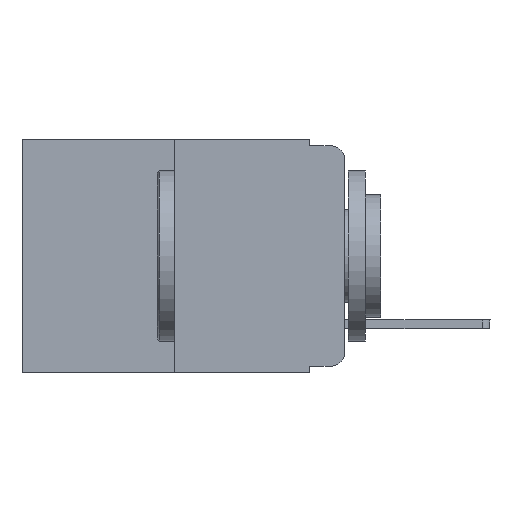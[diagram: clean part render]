
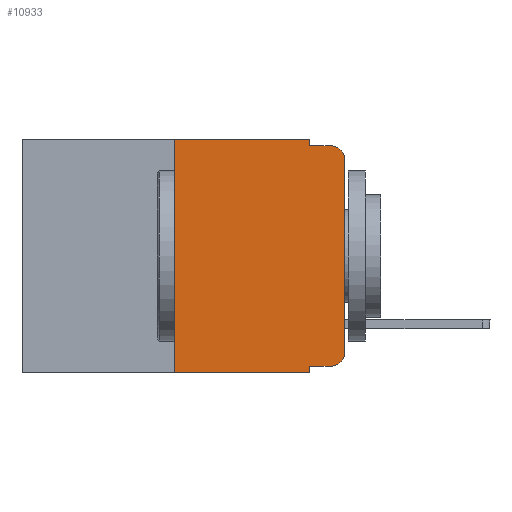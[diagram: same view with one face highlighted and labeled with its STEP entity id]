
A CAD part, left-side view. The second image highlights one B-rep face of the part: STEP entity #10933.
In plain terms, the highlighted planar face has unit normal (-1, 0, 0).
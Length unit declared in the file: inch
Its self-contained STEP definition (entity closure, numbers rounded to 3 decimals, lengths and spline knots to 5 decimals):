
#22 = CARTESIAN_POINT ( 'NONE',  ( 0., 0.051, -0.333 ) ) ;
#64 = DIRECTION ( 'NONE',  ( 0., 0., -1. ) ) ;
#146 = VECTOR ( 'NONE', #7066, 39.37008 ) ;
#222 = LINE ( 'NONE', #6759, #4909 ) ;
#269 = CARTESIAN_POINT ( 'NONE',  ( 0., 0.051, 0. ) ) ;
#316 = LINE ( 'NONE', #7918, #7166 ) ;
#426 = EDGE_CURVE ( 'NONE', #4306, #2158, #13773, .T. ) ;
#522 = CARTESIAN_POINT ( 'NONE',  ( 0., 0.02, -0.01 ) ) ;
#906 = CARTESIAN_POINT ( 'NONE',  ( 0., 0.25, 0. ) ) ;
#1368 = EDGE_LOOP ( 'NONE', ( #5111, #12547, #5237, #2367, #3803, #13229, #7071, #8952, #4279, #4212 ) ) ;
#1508 = VERTEX_POINT ( 'NONE', #906 ) ;
#1589 = LINE ( 'NONE', #14017, #3584 ) ;
#1869 = DIRECTION ( 'NONE',  ( -1., 0., 0. ) ) ;
#2158 = VERTEX_POINT ( 'NONE', #522 ) ;
#2354 = DIRECTION ( 'NONE',  ( 0., -1., 0. ) ) ;
#2367 = ORIENTED_EDGE ( 'NONE', *, *, #2426, .F. ) ;
#2403 = CIRCLE ( 'NONE', #7490, 0.02 ) ;
#2426 = EDGE_CURVE ( 'NONE', #7977, #4306, #222, .T. ) ;
#2478 = CARTESIAN_POINT ( 'NONE',  ( 0., 0., -0.03 ) ) ;
#2907 = DIRECTION ( 'NONE',  ( 0., 0., -1. ) ) ;
#3459 = LINE ( 'NONE', #269, #12423 ) ;
#3584 = VECTOR ( 'NONE', #5206, 39.37008 ) ;
#3803 = ORIENTED_EDGE ( 'NONE', *, *, #11077, .F. ) ;
#3999 = DIRECTION ( 'NONE',  ( 0., -1., 0. ) ) ;
#4024 = CARTESIAN_POINT ( 'NONE',  ( 0., 0.25, -0.343 ) ) ;
#4091 = EDGE_CURVE ( 'NONE', #8980, #8828, #10275, .T. ) ;
#4212 = ORIENTED_EDGE ( 'NONE', *, *, #5855, .T. ) ;
#4279 = ORIENTED_EDGE ( 'NONE', *, *, #4091, .T. ) ;
#4306 = VERTEX_POINT ( 'NONE', #5505 ) ;
#4570 = LINE ( 'NONE', #9970, #9867 ) ;
#4909 = VECTOR ( 'NONE', #64, 39.37008 ) ;
#5111 = ORIENTED_EDGE ( 'NONE', *, *, #8384, .T. ) ;
#5186 = VERTEX_POINT ( 'NONE', #2478 ) ;
#5206 = DIRECTION ( 'NONE',  ( 0., 0., 1. ) ) ;
#5237 = ORIENTED_EDGE ( 'NONE', *, *, #426, .F. ) ;
#5497 = AXIS2_PLACEMENT_3D ( 'NONE', #13297, #9700, #12213 ) ;
#5505 = CARTESIAN_POINT ( 'NONE',  ( 0., 0.051, -0.01 ) ) ;
#5759 = CARTESIAN_POINT ( 'NONE',  ( 0., 0.25, 0. ) ) ;
#5855 = EDGE_CURVE ( 'NONE', #8828, #12789, #2403, .T. ) ;
#6172 = CARTESIAN_POINT ( 'NONE',  ( 0., 0.051, -0.333 ) ) ;
#6341 = CARTESIAN_POINT ( 'NONE',  ( 0., 0., -0.313 ) ) ;
#6385 = DIRECTION ( 'NONE',  ( 1., 0., 0. ) ) ;
#6759 = CARTESIAN_POINT ( 'NONE',  ( 0., 0.051, 0. ) ) ;
#6895 = AXIS2_PLACEMENT_3D ( 'NONE', #10701, #6385, #2907 ) ;
#7066 = DIRECTION ( 'NONE',  ( 0., -1., 0. ) ) ;
#7071 = ORIENTED_EDGE ( 'NONE', *, *, #14133, .T. ) ;
#7166 = VECTOR ( 'NONE', #2354, 39.37008 ) ;
#7490 = AXIS2_PLACEMENT_3D ( 'NONE', #13669, #1869, #8530 ) ;
#7508 = EDGE_CURVE ( 'NONE', #12518, #1508, #7785, .T. ) ;
#7785 = LINE ( 'NONE', #5759, #12600 ) ;
#7918 = CARTESIAN_POINT ( 'NONE',  ( 0., 0.473, -0.343 ) ) ;
#7977 = VERTEX_POINT ( 'NONE', #9417 ) ;
#8284 = CARTESIAN_POINT ( 'NONE',  ( 0., 0.051, -0.01 ) ) ;
#8377 = VECTOR ( 'NONE', #3999, 39.37008 ) ;
#8384 = EDGE_CURVE ( 'NONE', #12789, #5186, #1589, .T. ) ;
#8530 = DIRECTION ( 'NONE',  ( 0., 0., -1. ) ) ;
#8538 = VERTEX_POINT ( 'NONE', #10906 ) ;
#8828 = VERTEX_POINT ( 'NONE', #12565 ) ;
#8952 = ORIENTED_EDGE ( 'NONE', *, *, #11555, .F. ) ;
#8980 = VERTEX_POINT ( 'NONE', #22 ) ;
#9417 = CARTESIAN_POINT ( 'NONE',  ( 0., 0.051, 0. ) ) ;
#9700 = DIRECTION ( 'NONE',  ( -1., 0., 0. ) ) ;
#9867 = VECTOR ( 'NONE', #14166, 39.37008 ) ;
#9970 = CARTESIAN_POINT ( 'NONE',  ( 0., 0.473, 0. ) ) ;
#10075 = DIRECTION ( 'NONE',  ( 0., 0., 1. ) ) ;
#10275 = LINE ( 'NONE', #6172, #8377 ) ;
#10701 = CARTESIAN_POINT ( 'NONE',  ( 0., 0.473, 0. ) ) ;
#10906 = CARTESIAN_POINT ( 'NONE',  ( 0., 0.051, -0.343 ) ) ;
#10933 = ADVANCED_FACE ( 'NONE', ( #14024 ), #14099, .F. ) ;
#11077 = EDGE_CURVE ( 'NONE', #1508, #7977, #4570, .T. ) ;
#11162 = EDGE_CURVE ( 'NONE', #5186, #2158, #13572, .T. ) ;
#11555 = EDGE_CURVE ( 'NONE', #8980, #8538, #3459, .T. ) ;
#12213 = DIRECTION ( 'NONE',  ( 0., 0., -1. ) ) ;
#12423 = VECTOR ( 'NONE', #12489, 39.37008 ) ;
#12489 = DIRECTION ( 'NONE',  ( 0., 0., -1. ) ) ;
#12518 = VERTEX_POINT ( 'NONE', #4024 ) ;
#12547 = ORIENTED_EDGE ( 'NONE', *, *, #11162, .T. ) ;
#12565 = CARTESIAN_POINT ( 'NONE',  ( 0., 0.02, -0.333 ) ) ;
#12600 = VECTOR ( 'NONE', #10075, 39.37008 ) ;
#12789 = VERTEX_POINT ( 'NONE', #6341 ) ;
#13229 = ORIENTED_EDGE ( 'NONE', *, *, #7508, .F. ) ;
#13297 = CARTESIAN_POINT ( 'NONE',  ( 0., 0.02, -0.03 ) ) ;
#13572 = CIRCLE ( 'NONE', #5497, 0.02 ) ;
#13669 = CARTESIAN_POINT ( 'NONE',  ( 0., 0.02, -0.313 ) ) ;
#13773 = LINE ( 'NONE', #8284, #146 ) ;
#14017 = CARTESIAN_POINT ( 'NONE',  ( 0., 0., 0. ) ) ;
#14024 = FACE_OUTER_BOUND ( 'NONE', #1368, .T. ) ;
#14099 = PLANE ( 'NONE',  #6895 ) ;
#14133 = EDGE_CURVE ( 'NONE', #12518, #8538, #316, .T. ) ;
#14166 = DIRECTION ( 'NONE',  ( 0., -1., 0. ) ) ;
